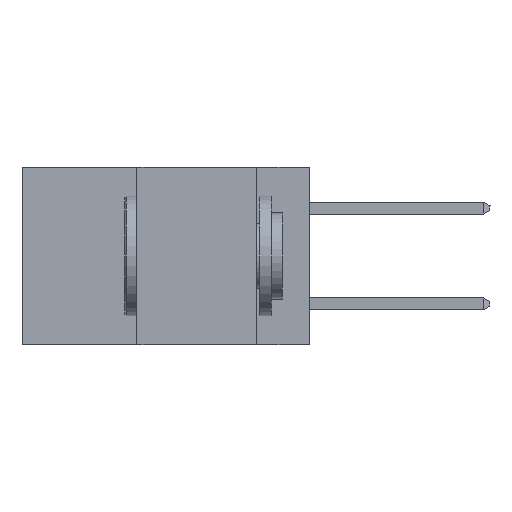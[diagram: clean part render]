
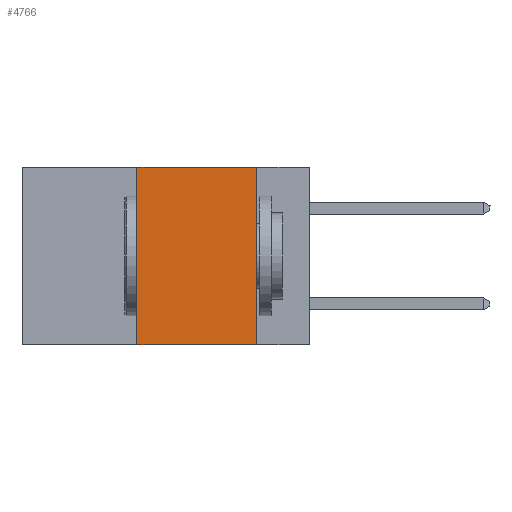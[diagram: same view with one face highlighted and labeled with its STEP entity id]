
A CAD part, left-side view. The second image highlights one B-rep face of the part: STEP entity #4766.
In plain terms, the highlighted planar face has unit normal (-1, 0, 0).
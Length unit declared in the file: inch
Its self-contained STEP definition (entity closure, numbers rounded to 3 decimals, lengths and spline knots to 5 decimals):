
#617 = VERTEX_POINT ( 'NONE', #8612 ) ;
#739 = DIRECTION ( 'NONE',  ( 1., 0., 0. ) ) ;
#976 = CARTESIAN_POINT ( 'NONE',  ( 0., 0.36, -0.37 ) ) ;
#995 = CARTESIAN_POINT ( 'NONE',  ( 0., 0.11, -0.37 ) ) ;
#1560 = PLANE ( 'NONE',  #10699 ) ;
#1914 = CARTESIAN_POINT ( 'NONE',  ( 0., 0.11, 0. ) ) ;
#1965 = VERTEX_POINT ( 'NONE', #7699 ) ;
#2004 = ORIENTED_EDGE ( 'NONE', *, *, #2646, .F. ) ;
#2159 = EDGE_LOOP ( 'NONE', ( #3468, #2004, #11462, #8272 ) ) ;
#2246 = VERTEX_POINT ( 'NONE', #995 ) ;
#2342 = LINE ( 'NONE', #6759, #11642 ) ;
#2376 = FACE_OUTER_BOUND ( 'NONE', #2159, .T. ) ;
#2646 = EDGE_CURVE ( 'NONE', #617, #1965, #8163, .T. ) ;
#2952 = VECTOR ( 'NONE', #9948, 39.37008 ) ;
#3468 = ORIENTED_EDGE ( 'NONE', *, *, #9713, .F. ) ;
#4229 = LINE ( 'NONE', #1914, #2952 ) ;
#4641 = VECTOR ( 'NONE', #9204, 39.37008 ) ;
#4727 = VECTOR ( 'NONE', #5704, 39.37008 ) ;
#4766 = ADVANCED_FACE ( 'NONE', ( #2376 ), #1560, .F. ) ;
#5236 = CARTESIAN_POINT ( 'NONE',  ( 0., 0.6, 0. ) ) ;
#5704 = DIRECTION ( 'NONE',  ( 0., -1., 0. ) ) ;
#5906 = DIRECTION ( 'NONE',  ( 0., 0., 1. ) ) ;
#6325 = EDGE_CURVE ( 'NONE', #6511, #617, #2342, .T. ) ;
#6511 = VERTEX_POINT ( 'NONE', #976 ) ;
#6759 = CARTESIAN_POINT ( 'NONE',  ( 0., 0.36, 0. ) ) ;
#6875 = EDGE_CURVE ( 'NONE', #6511, #2246, #7117, .T. ) ;
#7117 = LINE ( 'NONE', #7771, #4727 ) ;
#7699 = CARTESIAN_POINT ( 'NONE',  ( 0., 0.11, 0. ) ) ;
#7771 = CARTESIAN_POINT ( 'NONE',  ( 0., 0.6, -0.37 ) ) ;
#8163 = LINE ( 'NONE', #10018, #4641 ) ;
#8272 = ORIENTED_EDGE ( 'NONE', *, *, #6875, .T. ) ;
#8612 = CARTESIAN_POINT ( 'NONE',  ( 0., 0.36, 0. ) ) ;
#9204 = DIRECTION ( 'NONE',  ( 0., -1., 0. ) ) ;
#9713 = EDGE_CURVE ( 'NONE', #1965, #2246, #4229, .T. ) ;
#9718 = DIRECTION ( 'NONE',  ( 0., 0., -1. ) ) ;
#9948 = DIRECTION ( 'NONE',  ( 0., 0., -1. ) ) ;
#10018 = CARTESIAN_POINT ( 'NONE',  ( 0., 0.6, 0. ) ) ;
#10699 = AXIS2_PLACEMENT_3D ( 'NONE', #5236, #739, #9718 ) ;
#11462 = ORIENTED_EDGE ( 'NONE', *, *, #6325, .F. ) ;
#11642 = VECTOR ( 'NONE', #5906, 39.37008 ) ;
